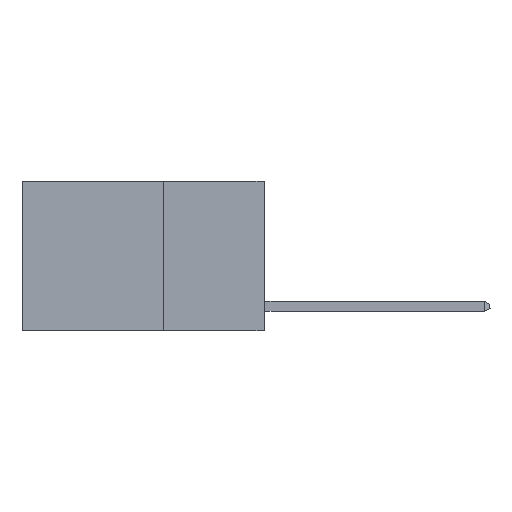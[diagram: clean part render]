
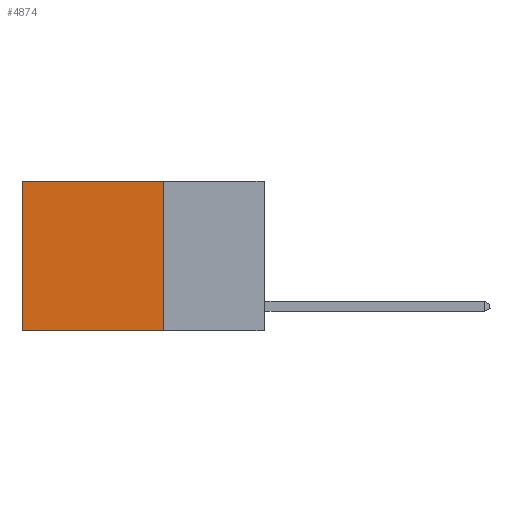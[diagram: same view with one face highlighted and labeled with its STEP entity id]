
A CAD part, left-side view. The second image highlights one B-rep face of the part: STEP entity #4874.
In plain terms, the highlighted planar face has unit normal (-1, 0, 0).
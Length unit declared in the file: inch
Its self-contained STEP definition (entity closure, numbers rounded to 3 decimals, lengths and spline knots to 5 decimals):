
#195 = EDGE_CURVE ( 'NONE', #1681, #13738, #878, .T. ) ;
#760 = DIRECTION ( 'NONE',  ( 0., 0., -1. ) ) ;
#805 = CARTESIAN_POINT ( 'NONE',  ( 0.2625, 0.25, 0. ) ) ;
#878 = LINE ( 'NONE', #4746, #8931 ) ;
#1681 = VERTEX_POINT ( 'NONE', #15079 ) ;
#2055 = AXIS2_PLACEMENT_3D ( 'NONE', #9370, #20463, #10990 ) ;
#2476 = DIRECTION ( 'NONE',  ( 0., 1., 0. ) ) ;
#3869 = EDGE_CURVE ( 'NONE', #18742, #1681, #10525, .T. ) ;
#4487 = FACE_OUTER_BOUND ( 'NONE', #9567, .T. ) ;
#4746 = CARTESIAN_POINT ( 'NONE',  ( 0.2625, 0.25, -0.37 ) ) ;
#4839 = CARTESIAN_POINT ( 'NONE',  ( 0.2625, 0.6, -0.37 ) ) ;
#4874 = ADVANCED_FACE ( 'NONE', ( #4487 ), #18827, .F. ) ;
#4879 = DIRECTION ( 'NONE',  ( 0., 1., 0. ) ) ;
#4884 = VERTEX_POINT ( 'NONE', #17157 ) ;
#5720 = CARTESIAN_POINT ( 'NONE',  ( 0.2625, 0.25, 0. ) ) ;
#5810 = CARTESIAN_POINT ( 'NONE',  ( 0.2625, 0.6, 0. ) ) ;
#6449 = ORIENTED_EDGE ( 'NONE', *, *, #15546, .T. ) ;
#6598 = ORIENTED_EDGE ( 'NONE', *, *, #18312, .T. ) ;
#7677 = ORIENTED_EDGE ( 'NONE', *, *, #195, .F. ) ;
#8414 = LINE ( 'NONE', #805, #20568 ) ;
#8931 = VECTOR ( 'NONE', #4879, 39.37008 ) ;
#9370 = CARTESIAN_POINT ( 'NONE',  ( 0.2625, 0.25, 0. ) ) ;
#9567 = EDGE_LOOP ( 'NONE', ( #6598, #7677, #10844, #6449 ) ) ;
#10525 = LINE ( 'NONE', #19876, #14168 ) ;
#10844 = ORIENTED_EDGE ( 'NONE', *, *, #3869, .F. ) ;
#10990 = DIRECTION ( 'NONE',  ( 0., 0., -1. ) ) ;
#13738 = VERTEX_POINT ( 'NONE', #4839 ) ;
#13833 = LINE ( 'NONE', #5810, #17495 ) ;
#14168 = VECTOR ( 'NONE', #760, 39.37008 ) ;
#15079 = CARTESIAN_POINT ( 'NONE',  ( 0.2625, 0.25, -0.37 ) ) ;
#15546 = EDGE_CURVE ( 'NONE', #18742, #4884, #8414, .T. ) ;
#17157 = CARTESIAN_POINT ( 'NONE',  ( 0.2625, 0.6, 0. ) ) ;
#17495 = VECTOR ( 'NONE', #18466, 39.37008 ) ;
#18312 = EDGE_CURVE ( 'NONE', #4884, #13738, #13833, .T. ) ;
#18466 = DIRECTION ( 'NONE',  ( 0., 0., -1. ) ) ;
#18742 = VERTEX_POINT ( 'NONE', #5720 ) ;
#18827 = PLANE ( 'NONE',  #2055 ) ;
#19876 = CARTESIAN_POINT ( 'NONE',  ( 0.2625, 0.25, 0. ) ) ;
#20463 = DIRECTION ( 'NONE',  ( 1., 0., 0. ) ) ;
#20568 = VECTOR ( 'NONE', #2476, 39.37008 ) ;
